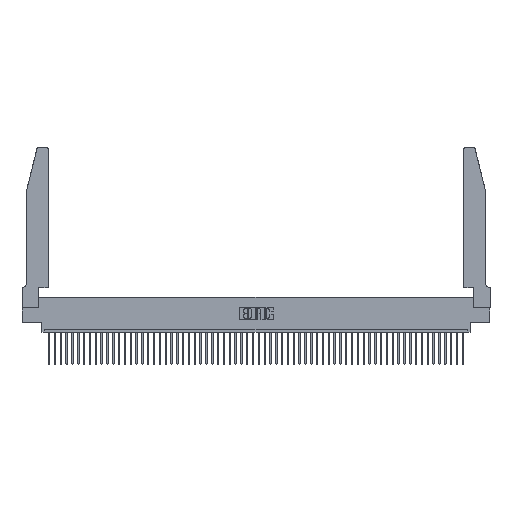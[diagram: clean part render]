
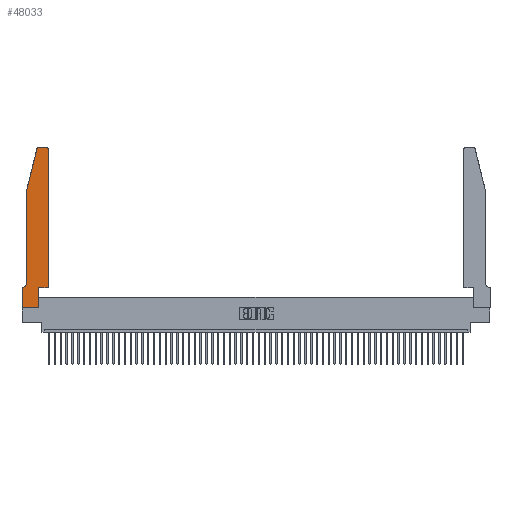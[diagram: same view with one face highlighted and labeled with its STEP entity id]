
A CAD part, top view. The second image highlights one B-rep face of the part: STEP entity #48033.
In plain terms, the highlighted planar face has unit normal (0, 0, 1).
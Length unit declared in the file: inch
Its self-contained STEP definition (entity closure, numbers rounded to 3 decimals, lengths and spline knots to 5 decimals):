
#147 = EDGE_CURVE ( 'NONE', #48215, #15207, #28887, .T. ) ;
#264 = ORIENTED_EDGE ( 'NONE', *, *, #30728, .T. ) ;
#1025 = DIRECTION ( 'NONE',  ( -1., 0., 0. ) ) ;
#1102 = CARTESIAN_POINT ( 'NONE',  ( 0.4505, 0.35, 0.37 ) ) ;
#1471 = AXIS2_PLACEMENT_3D ( 'NONE', #31296, #31478, #14487 ) ;
#1844 = EDGE_CURVE ( 'NONE', #9312, #52621, #37416, .T. ) ;
#2132 = VECTOR ( 'NONE', #24411, 39.37008 ) ;
#2619 = ORIENTED_EDGE ( 'NONE', *, *, #41364, .T. ) ;
#3054 = CARTESIAN_POINT ( 'NONE',  ( 0.4505, 0.35, 0.37 ) ) ;
#3542 = CARTESIAN_POINT ( 'NONE',  ( 0.0055, 0.35, 0.37 ) ) ;
#3699 = LINE ( 'NONE', #16877, #18313 ) ;
#4061 = CARTESIAN_POINT ( 'NONE',  ( 0., 0.35, 0.37 ) ) ;
#4294 = CARTESIAN_POINT ( 'NONE',  ( 0.25487, 2.72718, 0.37 ) ) ;
#4321 = CARTESIAN_POINT ( 'NONE',  ( 0., 0., 0.37 ) ) ;
#5963 = CARTESIAN_POINT ( 'NONE',  ( 0.284, 2.75, 0.37 ) ) ;
#6404 = DIRECTION ( 'NONE',  ( -1., 0., 0. ) ) ;
#7283 = LINE ( 'NONE', #28298, #27265 ) ;
#8108 = DIRECTION ( 'NONE',  ( 0., -1., 0. ) ) ;
#8190 = VERTEX_POINT ( 'NONE', #3542 ) ;
#8849 = DIRECTION ( 'NONE',  ( -1., 0., 0. ) ) ;
#9312 = VERTEX_POINT ( 'NONE', #36912 ) ;
#10699 = CARTESIAN_POINT ( 'NONE',  ( 0.2865, 0., 0.37 ) ) ;
#10804 = CARTESIAN_POINT ( 'NONE',  ( 0.0755, 0.35, 0.37 ) ) ;
#11735 = CIRCLE ( 'NONE', #36063, 0.03 ) ;
#11800 = EDGE_CURVE ( 'NONE', #20751, #8190, #32262, .T. ) ;
#11815 = CARTESIAN_POINT ( 'NONE',  ( 0.0755, 2., 0.37 ) ) ;
#12197 = DIRECTION ( 'NONE',  ( 1., 0., 0. ) ) ;
#12451 = ORIENTED_EDGE ( 'NONE', *, *, #1844, .T. ) ;
#12749 = DIRECTION ( 'NONE',  ( 0., 0., 1. ) ) ;
#12990 = FACE_OUTER_BOUND ( 'NONE', #49034, .T. ) ;
#14487 = DIRECTION ( 'NONE',  ( 1., 0., 0. ) ) ;
#15207 = VERTEX_POINT ( 'NONE', #3054 ) ;
#15857 = CARTESIAN_POINT ( 'NONE',  ( 0.4505, 0.35, 0.37 ) ) ;
#15911 = VERTEX_POINT ( 'NONE', #4294 ) ;
#16119 = ORIENTED_EDGE ( 'NONE', *, *, #147, .T. ) ;
#16169 = VERTEX_POINT ( 'NONE', #20035 ) ;
#16232 = AXIS2_PLACEMENT_3D ( 'NONE', #4061, #12749, #12197 ) ;
#16877 = CARTESIAN_POINT ( 'NONE',  ( 0.2605, 2.75, 0.37 ) ) ;
#17076 = CARTESIAN_POINT ( 'NONE',  ( 0.4205, 2.72, 0.37 ) ) ;
#17146 = EDGE_CURVE ( 'NONE', #28410, #15911, #42880, .T. ) ;
#17316 = VERTEX_POINT ( 'NONE', #40377 ) ;
#18138 = ORIENTED_EDGE ( 'NONE', *, *, #33308, .T. ) ;
#18313 = VECTOR ( 'NONE', #8849, 39.37008 ) ;
#18793 = LINE ( 'NONE', #1102, #32128 ) ;
#20035 = CARTESIAN_POINT ( 'NONE',  ( 0.4505, 2.72, 0.37 ) ) ;
#20751 = VERTEX_POINT ( 'NONE', #31040 ) ;
#22194 = CARTESIAN_POINT ( 'NONE',  ( 0.0055, 0.42, 0.37 ) ) ;
#22308 = CARTESIAN_POINT ( 'NONE',  ( 0., 0., 0.37 ) ) ;
#23307 = LINE ( 'NONE', #47390, #31340 ) ;
#24017 = DIRECTION ( 'NONE',  ( 0., 1., 0. ) ) ;
#24411 = DIRECTION ( 'NONE',  ( 0., -1., 0. ) ) ;
#26163 = LINE ( 'NONE', #10804, #36809 ) ;
#26189 = DIRECTION ( 'NONE',  ( 0., 0., 1. ) ) ;
#26351 = ORIENTED_EDGE ( 'NONE', *, *, #40518, .T. ) ;
#26479 = DIRECTION ( 'NONE',  ( 0., 0., -1. ) ) ;
#26890 = VECTOR ( 'NONE', #8108, 39.37008 ) ;
#27265 = VECTOR ( 'NONE', #24017, 39.37008 ) ;
#28298 = CARTESIAN_POINT ( 'NONE',  ( 0.2865, 0.35, 0.37 ) ) ;
#28410 = VERTEX_POINT ( 'NONE', #5963 ) ;
#28887 = LINE ( 'NONE', #15857, #36929 ) ;
#30494 = ORIENTED_EDGE ( 'NONE', *, *, #11800, .T. ) ;
#30728 = EDGE_CURVE ( 'NONE', #16169, #17316, #11735, .T. ) ;
#30854 = DIRECTION ( 'NONE',  ( 0., 1., 0. ) ) ;
#31040 = CARTESIAN_POINT ( 'NONE',  ( 0.0755, 0.42, 0.37 ) ) ;
#31296 = CARTESIAN_POINT ( 'NONE',  ( 0.284, 2.72, 0.37 ) ) ;
#31340 = VECTOR ( 'NONE', #33986, 39.37008 ) ;
#31478 = DIRECTION ( 'NONE',  ( 0., 0., 1. ) ) ;
#32128 = VECTOR ( 'NONE', #30854, 39.37008 ) ;
#32262 = CIRCLE ( 'NONE', #45875, 0.07 ) ;
#33308 = EDGE_CURVE ( 'NONE', #15207, #16169, #18793, .T. ) ;
#33568 = LINE ( 'NONE', #11815, #26890 ) ;
#33986 = DIRECTION ( 'NONE',  ( -0.239, -0.971, 0. ) ) ;
#34353 = ORIENTED_EDGE ( 'NONE', *, *, #47468, .T. ) ;
#34681 = EDGE_CURVE ( 'NONE', #40657, #48215, #7283, .T. ) ;
#35800 = ORIENTED_EDGE ( 'NONE', *, *, #45158, .T. ) ;
#36061 = CARTESIAN_POINT ( 'NONE',  ( 0.2865, 0.35, 0.37 ) ) ;
#36063 = AXIS2_PLACEMENT_3D ( 'NONE', #17076, #26189, #43346 ) ;
#36563 = DIRECTION ( 'NONE',  ( 1., 0., 0. ) ) ;
#36809 = VECTOR ( 'NONE', #6404, 39.37008 ) ;
#36912 = CARTESIAN_POINT ( 'NONE',  ( 0., 0.35, 0.37 ) ) ;
#36929 = VECTOR ( 'NONE', #36563, 39.37008 ) ;
#37416 = LINE ( 'NONE', #42281, #2132 ) ;
#37900 = VERTEX_POINT ( 'NONE', #43203 ) ;
#38289 = PLANE ( 'NONE',  #16232 ) ;
#39304 = ORIENTED_EDGE ( 'NONE', *, *, #34681, .T. ) ;
#40377 = CARTESIAN_POINT ( 'NONE',  ( 0.4205, 2.75, 0.37 ) ) ;
#40518 = EDGE_CURVE ( 'NONE', #17316, #28410, #3699, .T. ) ;
#40657 = VERTEX_POINT ( 'NONE', #10699 ) ;
#41364 = EDGE_CURVE ( 'NONE', #8190, #9312, #26163, .T. ) ;
#42281 = CARTESIAN_POINT ( 'NONE',  ( 0., 0., 0.37 ) ) ;
#42880 = CIRCLE ( 'NONE', #1471, 0.03 ) ;
#43018 = DIRECTION ( 'NONE',  ( 1., 0., 0. ) ) ;
#43203 = CARTESIAN_POINT ( 'NONE',  ( 0.0755, 2., 0.37 ) ) ;
#43346 = DIRECTION ( 'NONE',  ( 1., 0., 0. ) ) ;
#45158 = EDGE_CURVE ( 'NONE', #15911, #37900, #23307, .T. ) ;
#45875 = AXIS2_PLACEMENT_3D ( 'NONE', #22194, #26479, #1025 ) ;
#46345 = VECTOR ( 'NONE', #43018, 39.37008 ) ;
#47390 = CARTESIAN_POINT ( 'NONE',  ( 0.0755, 2., 0.37 ) ) ;
#47468 = EDGE_CURVE ( 'NONE', #52621, #40657, #51000, .T. ) ;
#48033 = ADVANCED_FACE ( 'NONE', ( #12990 ), #38289, .T. ) ;
#48215 = VERTEX_POINT ( 'NONE', #36061 ) ;
#49034 = EDGE_LOOP ( 'NONE', ( #26351, #51339, #35800, #49812, #30494, #2619, #12451, #34353, #39304, #16119, #18138, #264 ) ) ;
#49812 = ORIENTED_EDGE ( 'NONE', *, *, #54935, .T. ) ;
#51000 = LINE ( 'NONE', #4321, #46345 ) ;
#51339 = ORIENTED_EDGE ( 'NONE', *, *, #17146, .T. ) ;
#52621 = VERTEX_POINT ( 'NONE', #22308 ) ;
#54935 = EDGE_CURVE ( 'NONE', #37900, #20751, #33568, .T. ) ;
